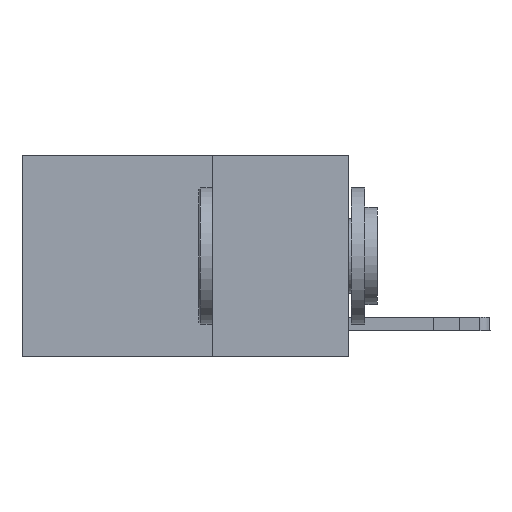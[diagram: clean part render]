
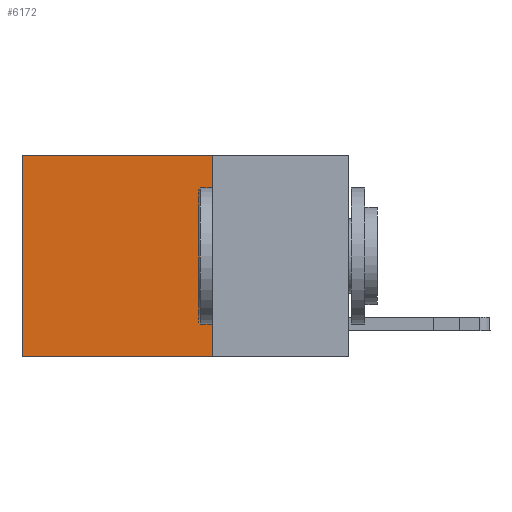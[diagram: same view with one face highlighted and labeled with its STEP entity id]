
A CAD part, left-side view. The second image highlights one B-rep face of the part: STEP entity #6172.
In plain terms, the highlighted planar face has unit normal (-1, 0, 0).
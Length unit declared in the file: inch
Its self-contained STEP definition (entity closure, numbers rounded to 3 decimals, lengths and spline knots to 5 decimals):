
#1 = VECTOR ( 'NONE', #19890, 39.37008 ) ;
#538 = DIRECTION ( 'NONE',  ( 0., 0., -1. ) ) ;
#998 = LINE ( 'NONE', #15872, #3752 ) ;
#1714 = EDGE_CURVE ( 'NONE', #23204, #5623, #2938, .T. ) ;
#1954 = EDGE_LOOP ( 'NONE', ( #23242, #10071, #5253, #17482 ) ) ;
#2513 = VECTOR ( 'NONE', #10133, 39.37008 ) ;
#2938 = LINE ( 'NONE', #11856, #2513 ) ;
#3720 = DIRECTION ( 'NONE',  ( 0., 0., -1. ) ) ;
#3752 = VECTOR ( 'NONE', #538, 39.37008 ) ;
#4971 = CARTESIAN_POINT ( 'NONE',  ( 0.2625, 0.25, 0. ) ) ;
#5222 = DIRECTION ( 'NONE',  ( 1., 0., 0. ) ) ;
#5253 = ORIENTED_EDGE ( 'NONE', *, *, #5805, .F. ) ;
#5571 = PLANE ( 'NONE',  #8584 ) ;
#5623 = VERTEX_POINT ( 'NONE', #22984 ) ;
#5805 = EDGE_CURVE ( 'NONE', #19543, #23204, #998, .T. ) ;
#5953 = CARTESIAN_POINT ( 'NONE',  ( 0.2625, 0.25, -0.37 ) ) ;
#6172 = ADVANCED_FACE ( 'NONE', ( #22324 ), #5571, .F. ) ;
#8584 = AXIS2_PLACEMENT_3D ( 'NONE', #12983, #5222, #18285 ) ;
#10071 = ORIENTED_EDGE ( 'NONE', *, *, #1714, .F. ) ;
#10133 = DIRECTION ( 'NONE',  ( 0., 1., 0. ) ) ;
#10653 = EDGE_CURVE ( 'NONE', #20751, #5623, #14771, .T. ) ;
#11856 = CARTESIAN_POINT ( 'NONE',  ( 0.2625, 0.25, -0.37 ) ) ;
#12780 = CARTESIAN_POINT ( 'NONE',  ( 0.2625, 0.25, 0. ) ) ;
#12983 = CARTESIAN_POINT ( 'NONE',  ( 0.2625, 0.25, 0. ) ) ;
#13511 = VECTOR ( 'NONE', #3720, 39.37008 ) ;
#14273 = EDGE_CURVE ( 'NONE', #19543, #20751, #21731, .T. ) ;
#14771 = LINE ( 'NONE', #16517, #13511 ) ;
#15872 = CARTESIAN_POINT ( 'NONE',  ( 0.2625, 0.25, 0. ) ) ;
#16417 = CARTESIAN_POINT ( 'NONE',  ( 0.2625, 0.6, 0. ) ) ;
#16517 = CARTESIAN_POINT ( 'NONE',  ( 0.2625, 0.6, 0. ) ) ;
#17482 = ORIENTED_EDGE ( 'NONE', *, *, #14273, .T. ) ;
#18285 = DIRECTION ( 'NONE',  ( 0., 0., -1. ) ) ;
#19543 = VERTEX_POINT ( 'NONE', #12780 ) ;
#19890 = DIRECTION ( 'NONE',  ( 0., 1., 0. ) ) ;
#20751 = VERTEX_POINT ( 'NONE', #16417 ) ;
#21731 = LINE ( 'NONE', #4971, #1 ) ;
#22324 = FACE_OUTER_BOUND ( 'NONE', #1954, .T. ) ;
#22984 = CARTESIAN_POINT ( 'NONE',  ( 0.2625, 0.6, -0.37 ) ) ;
#23204 = VERTEX_POINT ( 'NONE', #5953 ) ;
#23242 = ORIENTED_EDGE ( 'NONE', *, *, #10653, .T. ) ;
